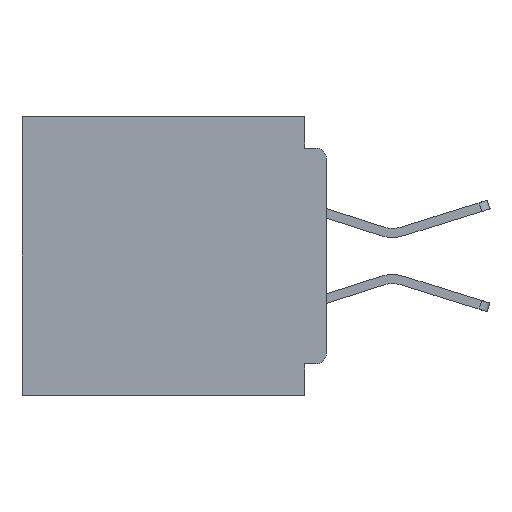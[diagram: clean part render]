
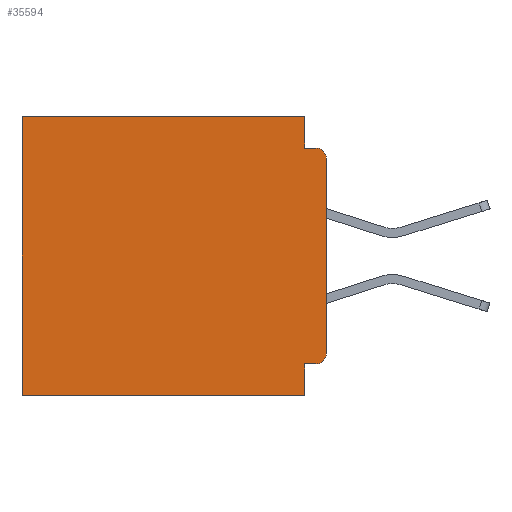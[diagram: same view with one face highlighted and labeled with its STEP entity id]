
A CAD part, left-side view. The second image highlights one B-rep face of the part: STEP entity #35594.
In plain terms, the highlighted planar face has unit normal (-1, 0, 0).
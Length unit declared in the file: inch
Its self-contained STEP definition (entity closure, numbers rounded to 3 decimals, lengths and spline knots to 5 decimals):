
#170 = DIRECTION ( 'NONE',  ( 0., 0., -1. ) ) ;
#306 = AXIS2_PLACEMENT_3D ( 'NONE', #23323, #7873, #29496 ) ;
#987 = DIRECTION ( 'NONE',  ( 0., 1., 0. ) ) ;
#2026 = LINE ( 'NONE', #35709, #10277 ) ;
#2254 = LINE ( 'NONE', #4566, #17754 ) ;
#2843 = FACE_OUTER_BOUND ( 'NONE', #9415, .T. ) ;
#3240 = VERTEX_POINT ( 'NONE', #28616 ) ;
#3369 = LINE ( 'NONE', #28742, #35164 ) ;
#3987 = EDGE_CURVE ( 'NONE', #21752, #3240, #37644, .T. ) ;
#4035 = VERTEX_POINT ( 'NONE', #11412 ) ;
#4074 = ORIENTED_EDGE ( 'NONE', *, *, #26790, .F. ) ;
#4254 = ORIENTED_EDGE ( 'NONE', *, *, #22400, .T. ) ;
#4566 = CARTESIAN_POINT ( 'NONE',  ( 0.3, 0., -0.355 ) ) ;
#4826 = CARTESIAN_POINT ( 'NONE',  ( 0.3, 0.031, 0. ) ) ;
#5025 = VECTOR ( 'NONE', #38507, 39.37008 ) ;
#5633 = DIRECTION ( 'NONE',  ( -1., 0., 0. ) ) ;
#5719 = DIRECTION ( 'NONE',  ( 0., 0., -1. ) ) ;
#6861 = ORIENTED_EDGE ( 'NONE', *, *, #3987, .T. ) ;
#7023 = AXIS2_PLACEMENT_3D ( 'NONE', #31300, #12897, #34348 ) ;
#7363 = CARTESIAN_POINT ( 'NONE',  ( 0.3, 0.015, -0.34 ) ) ;
#7873 = DIRECTION ( 'NONE',  ( 1., 0., 0. ) ) ;
#7984 = VECTOR ( 'NONE', #15006, 39.37008 ) ;
#8076 = ORIENTED_EDGE ( 'NONE', *, *, #32085, .F. ) ;
#8135 = AXIS2_PLACEMENT_3D ( 'NONE', #7363, #5633, #5719 ) ;
#9415 = EDGE_LOOP ( 'NONE', ( #24205, #35559, #4074, #8076, #4254, #34564, #21333, #9909, #25285, #6861 ) ) ;
#9909 = ORIENTED_EDGE ( 'NONE', *, *, #15491, .F. ) ;
#10277 = VECTOR ( 'NONE', #23448, 39.37008 ) ;
#11015 = CARTESIAN_POINT ( 'NONE',  ( 0.3, 0., -0.045 ) ) ;
#11138 = EDGE_CURVE ( 'NONE', #21752, #4035, #2254, .T. ) ;
#11203 = VERTEX_POINT ( 'NONE', #4826 ) ;
#11412 = CARTESIAN_POINT ( 'NONE',  ( 0.3, 0.031, -0.355 ) ) ;
#12051 = DIRECTION ( 'NONE',  ( 0., 0., -1. ) ) ;
#12897 = DIRECTION ( 'NONE',  ( -1., 0., 0. ) ) ;
#13296 = LINE ( 'NONE', #11015, #5025 ) ;
#13578 = LINE ( 'NONE', #37122, #29018 ) ;
#14529 = EDGE_CURVE ( 'NONE', #18381, #36800, #2026, .T. ) ;
#14909 = DIRECTION ( 'NONE',  ( 0., 0., -1. ) ) ;
#15006 = DIRECTION ( 'NONE',  ( 0., 1., 0. ) ) ;
#15491 = EDGE_CURVE ( 'NONE', #4035, #37458, #13578, .T. ) ;
#16343 = CARTESIAN_POINT ( 'NONE',  ( 0.3, 0.015, -0.045 ) ) ;
#17035 = DIRECTION ( 'NONE',  ( 0., 1., 0. ) ) ;
#17754 = VECTOR ( 'NONE', #17035, 39.37008 ) ;
#18381 = VERTEX_POINT ( 'NONE', #34450 ) ;
#18811 = EDGE_CURVE ( 'NONE', #37458, #36800, #31602, .T. ) ;
#19375 = VERTEX_POINT ( 'NONE', #27196 ) ;
#20212 = LINE ( 'NONE', #30356, #36494 ) ;
#20813 = CARTESIAN_POINT ( 'NONE',  ( 0.3, 0.031, -0.4 ) ) ;
#21333 = ORIENTED_EDGE ( 'NONE', *, *, #18811, .F. ) ;
#21752 = VERTEX_POINT ( 'NONE', #28792 ) ;
#22400 = EDGE_CURVE ( 'NONE', #11203, #18381, #3369, .T. ) ;
#23323 = CARTESIAN_POINT ( 'NONE',  ( 0.3, 0., -0.4 ) ) ;
#23448 = DIRECTION ( 'NONE',  ( 0., 0., -1. ) ) ;
#23823 = VERTEX_POINT ( 'NONE', #29021 ) ;
#24205 = ORIENTED_EDGE ( 'NONE', *, *, #36472, .F. ) ;
#24983 = EDGE_CURVE ( 'NONE', #19375, #27925, #32126, .T. ) ;
#25285 = ORIENTED_EDGE ( 'NONE', *, *, #11138, .F. ) ;
#26403 = PLANE ( 'NONE',  #306 ) ;
#26790 = EDGE_CURVE ( 'NONE', #23823, #27925, #13296, .T. ) ;
#27196 = CARTESIAN_POINT ( 'NONE',  ( 0.3, 0., -0.06 ) ) ;
#27925 = VERTEX_POINT ( 'NONE', #16343 ) ;
#28616 = CARTESIAN_POINT ( 'NONE',  ( 0.3, 0., -0.34 ) ) ;
#28742 = CARTESIAN_POINT ( 'NONE',  ( 0.3, 0., 0. ) ) ;
#28792 = CARTESIAN_POINT ( 'NONE',  ( 0.3, 0.015, -0.355 ) ) ;
#29018 = VECTOR ( 'NONE', #170, 39.37008 ) ;
#29021 = CARTESIAN_POINT ( 'NONE',  ( 0.3, 0.031, -0.045 ) ) ;
#29127 = CARTESIAN_POINT ( 'NONE',  ( 0.3, 0.437, -0.4 ) ) ;
#29496 = DIRECTION ( 'NONE',  ( 0., 0., -1. ) ) ;
#30356 = CARTESIAN_POINT ( 'NONE',  ( 0.3, 0., -0.4 ) ) ;
#30747 = VECTOR ( 'NONE', #14909, 39.37008 ) ;
#31300 = CARTESIAN_POINT ( 'NONE',  ( 0.3, 0.015, -0.06 ) ) ;
#31602 = LINE ( 'NONE', #36441, #7984 ) ;
#32085 = EDGE_CURVE ( 'NONE', #11203, #23823, #37870, .T. ) ;
#32126 = CIRCLE ( 'NONE', #7023, 0.015 ) ;
#33264 = CARTESIAN_POINT ( 'NONE',  ( 0.3, 0.031, 0. ) ) ;
#34348 = DIRECTION ( 'NONE',  ( 0., 0., -1. ) ) ;
#34450 = CARTESIAN_POINT ( 'NONE',  ( 0.3, 0.437, 0. ) ) ;
#34564 = ORIENTED_EDGE ( 'NONE', *, *, #14529, .T. ) ;
#35164 = VECTOR ( 'NONE', #987, 39.37008 ) ;
#35559 = ORIENTED_EDGE ( 'NONE', *, *, #24983, .T. ) ;
#35594 = ADVANCED_FACE ( 'NONE', ( #2843 ), #26403, .F. ) ;
#35709 = CARTESIAN_POINT ( 'NONE',  ( 0.3, 0.437, -0.4 ) ) ;
#36441 = CARTESIAN_POINT ( 'NONE',  ( 0.3, 0., -0.4 ) ) ;
#36472 = EDGE_CURVE ( 'NONE', #19375, #3240, #20212, .T. ) ;
#36494 = VECTOR ( 'NONE', #12051, 39.37008 ) ;
#36800 = VERTEX_POINT ( 'NONE', #29127 ) ;
#37122 = CARTESIAN_POINT ( 'NONE',  ( 0.3, 0.031, -0.4 ) ) ;
#37458 = VERTEX_POINT ( 'NONE', #20813 ) ;
#37644 = CIRCLE ( 'NONE', #8135, 0.015 ) ;
#37870 = LINE ( 'NONE', #33264, #30747 ) ;
#38507 = DIRECTION ( 'NONE',  ( 0., -1., 0. ) ) ;
